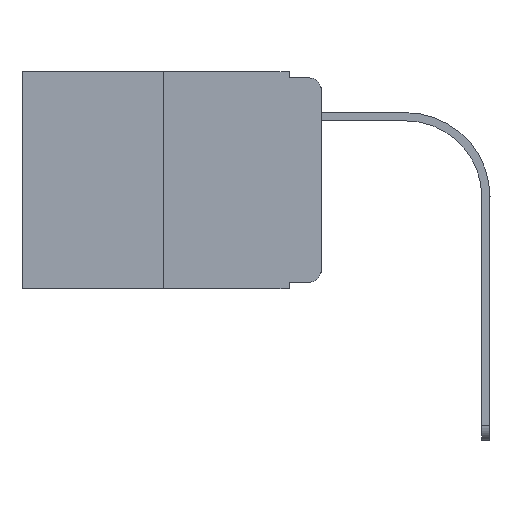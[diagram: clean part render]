
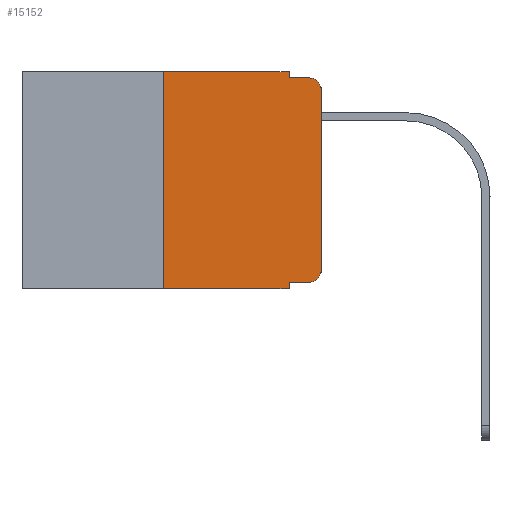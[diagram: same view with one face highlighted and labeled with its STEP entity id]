
A CAD part, left-side view. The second image highlights one B-rep face of the part: STEP entity #15152.
In plain terms, the highlighted planar face has unit normal (-1, 0, 0).
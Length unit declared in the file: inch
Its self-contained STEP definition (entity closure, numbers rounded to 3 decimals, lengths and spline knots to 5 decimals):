
#247 = CARTESIAN_POINT ( 'NONE',  ( 0., 0.02, -0.01 ) ) ;
#486 = DIRECTION ( 'NONE',  ( 0., 0., -1. ) ) ;
#519 = LINE ( 'NONE', #11107, #7363 ) ;
#655 = VERTEX_POINT ( 'NONE', #19134 ) ;
#699 = VECTOR ( 'NONE', #10246, 39.37008 ) ;
#715 = EDGE_CURVE ( 'NONE', #10972, #11194, #14017, .T. ) ;
#1205 = DIRECTION ( 'NONE',  ( 0., 0., -1. ) ) ;
#1207 = CARTESIAN_POINT ( 'NONE',  ( 0., 0.473, -0.343 ) ) ;
#1556 = VERTEX_POINT ( 'NONE', #17379 ) ;
#1629 = DIRECTION ( 'NONE',  ( 1., 0., 0. ) ) ;
#1896 = VERTEX_POINT ( 'NONE', #18848 ) ;
#2056 = VECTOR ( 'NONE', #2741, 39.37008 ) ;
#2444 = DIRECTION ( 'NONE',  ( 0., -1., 0. ) ) ;
#2741 = DIRECTION ( 'NONE',  ( 0., -1., 0. ) ) ;
#2851 = CARTESIAN_POINT ( 'NONE',  ( 0., 0.473, 0. ) ) ;
#3801 = ORIENTED_EDGE ( 'NONE', *, *, #13162, .F. ) ;
#4864 = ORIENTED_EDGE ( 'NONE', *, *, #6329, .T. ) ;
#5515 = VERTEX_POINT ( 'NONE', #9851 ) ;
#5543 = DIRECTION ( 'NONE',  ( 0., 0., 1. ) ) ;
#5740 = ORIENTED_EDGE ( 'NONE', *, *, #14411, .F. ) ;
#5816 = ORIENTED_EDGE ( 'NONE', *, *, #715, .F. ) ;
#5919 = EDGE_LOOP ( 'NONE', ( #11819, #21078, #5740, #15922, #5816, #12081, #12981, #3801, #8471, #4864 ) ) ;
#6033 = CARTESIAN_POINT ( 'NONE',  ( 0., 0.051, 0. ) ) ;
#6244 = PLANE ( 'NONE',  #20520 ) ;
#6302 = VERTEX_POINT ( 'NONE', #247 ) ;
#6329 = EDGE_CURVE ( 'NONE', #1896, #12965, #17594, .T. ) ;
#6349 = DIRECTION ( 'NONE',  ( 0., 0., -1. ) ) ;
#7112 = EDGE_CURVE ( 'NONE', #12965, #19549, #519, .T. ) ;
#7363 = VECTOR ( 'NONE', #5543, 39.37008 ) ;
#7967 = LINE ( 'NONE', #6033, #12986 ) ;
#7983 = EDGE_CURVE ( 'NONE', #5515, #10972, #14291, .T. ) ;
#8303 = CARTESIAN_POINT ( 'NONE',  ( 0., 0.051, -0.01 ) ) ;
#8471 = ORIENTED_EDGE ( 'NONE', *, *, #14647, .T. ) ;
#8650 = LINE ( 'NONE', #15191, #17458 ) ;
#8884 = CARTESIAN_POINT ( 'NONE',  ( 0., 0.051, -0.333 ) ) ;
#9723 = AXIS2_PLACEMENT_3D ( 'NONE', #13658, #18357, #20056 ) ;
#9781 = CARTESIAN_POINT ( 'NONE',  ( 0., 0.473, 0. ) ) ;
#9851 = CARTESIAN_POINT ( 'NONE',  ( 0., 0.25, -0.343 ) ) ;
#9926 = VECTOR ( 'NONE', #2444, 39.37008 ) ;
#10246 = DIRECTION ( 'NONE',  ( 0., -1., 0. ) ) ;
#10674 = VERTEX_POINT ( 'NONE', #15588 ) ;
#10972 = VERTEX_POINT ( 'NONE', #19815 ) ;
#11107 = CARTESIAN_POINT ( 'NONE',  ( 0., 0., 0. ) ) ;
#11194 = VERTEX_POINT ( 'NONE', #20653 ) ;
#11369 = DIRECTION ( 'NONE',  ( 0., 0., 1. ) ) ;
#11819 = ORIENTED_EDGE ( 'NONE', *, *, #7112, .T. ) ;
#11998 = LINE ( 'NONE', #8884, #9926 ) ;
#12032 = DIRECTION ( 'NONE',  ( -1., 0., 0. ) ) ;
#12081 = ORIENTED_EDGE ( 'NONE', *, *, #7983, .F. ) ;
#12828 = VECTOR ( 'NONE', #11369, 39.37008 ) ;
#12965 = VERTEX_POINT ( 'NONE', #14768 ) ;
#12981 = ORIENTED_EDGE ( 'NONE', *, *, #15043, .T. ) ;
#12986 = VECTOR ( 'NONE', #1205, 39.37008 ) ;
#13129 = LINE ( 'NONE', #8303, #15058 ) ;
#13162 = EDGE_CURVE ( 'NONE', #1556, #10674, #8650, .T. ) ;
#13658 = CARTESIAN_POINT ( 'NONE',  ( 0., 0.02, -0.313 ) ) ;
#13816 = EDGE_CURVE ( 'NONE', #11194, #655, #7967, .T. ) ;
#14017 = LINE ( 'NONE', #2851, #2056 ) ;
#14291 = LINE ( 'NONE', #17593, #12828 ) ;
#14411 = EDGE_CURVE ( 'NONE', #655, #6302, #13129, .T. ) ;
#14647 = EDGE_CURVE ( 'NONE', #1556, #1896, #11998, .T. ) ;
#14768 = CARTESIAN_POINT ( 'NONE',  ( 0., 0., -0.313 ) ) ;
#15043 = EDGE_CURVE ( 'NONE', #5515, #10674, #20794, .T. ) ;
#15058 = VECTOR ( 'NONE', #19841, 39.37008 ) ;
#15152 = ADVANCED_FACE ( 'NONE', ( #19622 ), #6244, .F. ) ;
#15191 = CARTESIAN_POINT ( 'NONE',  ( 0., 0.051, 0. ) ) ;
#15251 = DIRECTION ( 'NONE',  ( 0., 0., -1. ) ) ;
#15372 = EDGE_CURVE ( 'NONE', #19549, #6302, #15456, .T. ) ;
#15456 = CIRCLE ( 'NONE', #20884, 0.02 ) ;
#15588 = CARTESIAN_POINT ( 'NONE',  ( 0., 0.051, -0.343 ) ) ;
#15922 = ORIENTED_EDGE ( 'NONE', *, *, #13816, .F. ) ;
#17379 = CARTESIAN_POINT ( 'NONE',  ( 0., 0.051, -0.333 ) ) ;
#17458 = VECTOR ( 'NONE', #486, 39.37008 ) ;
#17593 = CARTESIAN_POINT ( 'NONE',  ( 0., 0.25, 0. ) ) ;
#17594 = CIRCLE ( 'NONE', #9723, 0.02 ) ;
#18072 = CARTESIAN_POINT ( 'NONE',  ( 0., 0., -0.03 ) ) ;
#18233 = CARTESIAN_POINT ( 'NONE',  ( 0., 0.02, -0.03 ) ) ;
#18357 = DIRECTION ( 'NONE',  ( -1., 0., 0. ) ) ;
#18848 = CARTESIAN_POINT ( 'NONE',  ( 0., 0.02, -0.333 ) ) ;
#19134 = CARTESIAN_POINT ( 'NONE',  ( 0., 0.051, -0.01 ) ) ;
#19549 = VERTEX_POINT ( 'NONE', #18072 ) ;
#19622 = FACE_OUTER_BOUND ( 'NONE', #5919, .T. ) ;
#19815 = CARTESIAN_POINT ( 'NONE',  ( 0., 0.25, 0. ) ) ;
#19841 = DIRECTION ( 'NONE',  ( 0., -1., 0. ) ) ;
#20056 = DIRECTION ( 'NONE',  ( 0., 0., -1. ) ) ;
#20520 = AXIS2_PLACEMENT_3D ( 'NONE', #9781, #1629, #6349 ) ;
#20653 = CARTESIAN_POINT ( 'NONE',  ( 0., 0.051, 0. ) ) ;
#20794 = LINE ( 'NONE', #1207, #699 ) ;
#20884 = AXIS2_PLACEMENT_3D ( 'NONE', #18233, #12032, #15251 ) ;
#21078 = ORIENTED_EDGE ( 'NONE', *, *, #15372, .T. ) ;
